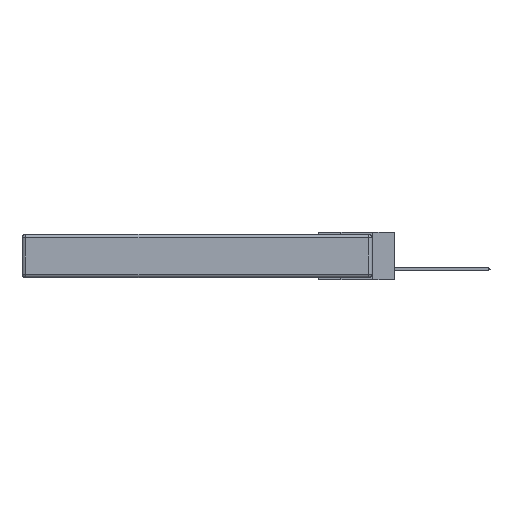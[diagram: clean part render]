
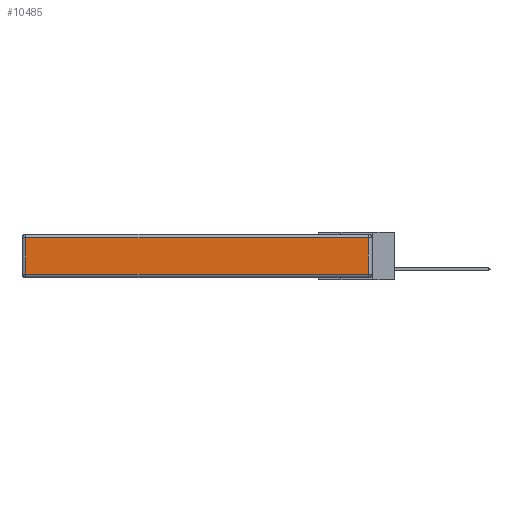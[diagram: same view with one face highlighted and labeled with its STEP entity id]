
A CAD part, left-side view. The second image highlights one B-rep face of the part: STEP entity #10485.
In plain terms, the highlighted planar face has unit normal (-1, 0, 0).
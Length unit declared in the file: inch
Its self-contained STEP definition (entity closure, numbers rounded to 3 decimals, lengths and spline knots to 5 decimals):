
#195 = LINE ( 'NONE', #5162, #11475 ) ;
#400 = CARTESIAN_POINT ( 'NONE',  ( 0., 0.03, -0.343 ) ) ;
#854 = ORIENTED_EDGE ( 'NONE', *, *, #10496, .T. ) ;
#990 = CARTESIAN_POINT ( 'NONE',  ( 0., 2.72, -0.03 ) ) ;
#1737 = CARTESIAN_POINT ( 'NONE',  ( 0., 0., -0.343 ) ) ;
#3333 = VECTOR ( 'NONE', #17300, 39.37008 ) ;
#3700 = CARTESIAN_POINT ( 'NONE',  ( 0., 0.03, -0.313 ) ) ;
#5003 = PLANE ( 'NONE',  #16753 ) ;
#5088 = CARTESIAN_POINT ( 'NONE',  ( 0., 2.75, -0.03 ) ) ;
#5162 = CARTESIAN_POINT ( 'NONE',  ( 0., 0., -0.313 ) ) ;
#5588 = CARTESIAN_POINT ( 'NONE',  ( 0., 2.72, -0.343 ) ) ;
#5849 = CARTESIAN_POINT ( 'NONE',  ( 0., 2.72, -0.313 ) ) ;
#5914 = LINE ( 'NONE', #5588, #14805 ) ;
#8437 = FACE_OUTER_BOUND ( 'NONE', #18271, .T. ) ;
#8941 = ORIENTED_EDGE ( 'NONE', *, *, #15602, .T. ) ;
#10337 = LINE ( 'NONE', #5088, #3333 ) ;
#10485 = ADVANCED_FACE ( 'NONE', ( #8437 ), #5003, .T. ) ;
#10496 = EDGE_CURVE ( 'NONE', #16005, #19299, #10337, .T. ) ;
#10935 = ORIENTED_EDGE ( 'NONE', *, *, #14170, .T. ) ;
#11164 = EDGE_CURVE ( 'NONE', #13399, #16005, #14048, .T. ) ;
#11475 = VECTOR ( 'NONE', #15489, 39.37008 ) ;
#12940 = CARTESIAN_POINT ( 'NONE',  ( 0., 0.03, -0.03 ) ) ;
#13399 = VERTEX_POINT ( 'NONE', #3700 ) ;
#13844 = ORIENTED_EDGE ( 'NONE', *, *, #11164, .T. ) ;
#14048 = LINE ( 'NONE', #400, #16775 ) ;
#14170 = EDGE_CURVE ( 'NONE', #19299, #19106, #5914, .T. ) ;
#14805 = VECTOR ( 'NONE', #19568, 39.37008 ) ;
#15489 = DIRECTION ( 'NONE',  ( 0., -1., 0. ) ) ;
#15602 = EDGE_CURVE ( 'NONE', #19106, #13399, #195, .T. ) ;
#15708 = DIRECTION ( 'NONE',  ( -1., 0., 0. ) ) ;
#15954 = DIRECTION ( 'NONE',  ( 0., 0., 1. ) ) ;
#16005 = VERTEX_POINT ( 'NONE', #12940 ) ;
#16753 = AXIS2_PLACEMENT_3D ( 'NONE', #1737, #15708, #20723 ) ;
#16775 = VECTOR ( 'NONE', #15954, 39.37008 ) ;
#17300 = DIRECTION ( 'NONE',  ( 0., 1., 0. ) ) ;
#18271 = EDGE_LOOP ( 'NONE', ( #8941, #13844, #854, #10935 ) ) ;
#19106 = VERTEX_POINT ( 'NONE', #5849 ) ;
#19299 = VERTEX_POINT ( 'NONE', #990 ) ;
#19568 = DIRECTION ( 'NONE',  ( 0., 0., -1. ) ) ;
#20723 = DIRECTION ( 'NONE',  ( 0., 0., 1. ) ) ;
